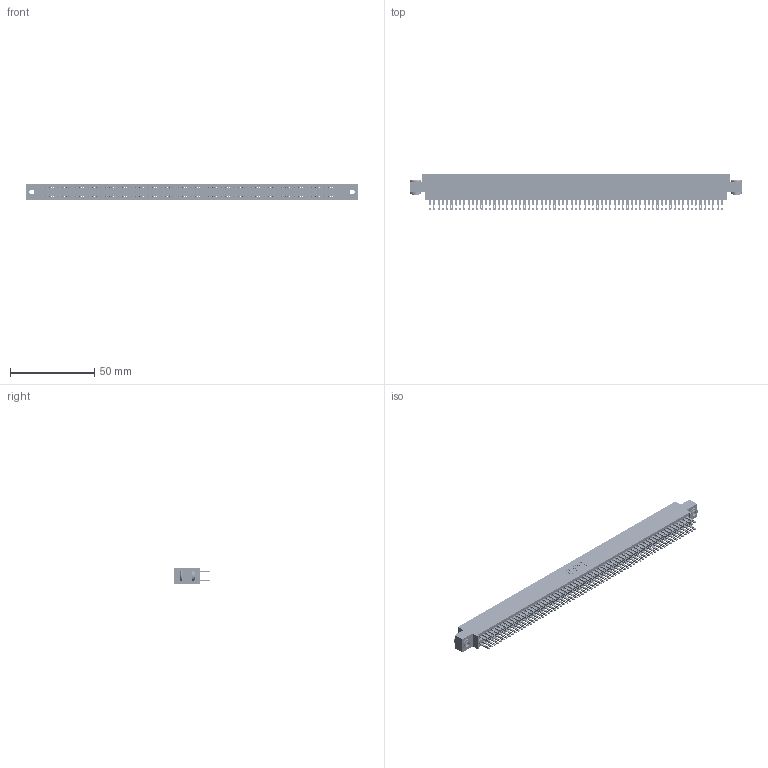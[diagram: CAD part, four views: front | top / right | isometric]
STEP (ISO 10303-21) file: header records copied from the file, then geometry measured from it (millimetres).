
FILE_DESCRIPTION (( 'STEP AP203' ), '1' );
FILE_NAME ('895-138-500-803.STEP', '2020-10-13T19:05:36', ( '' ), ( '' ), 'SwSTEP 2.0', 'SolidWorks 2020', '' );
FILE_SCHEMA (( 'CONFIG_CONTROL_DESIGN' ));
Length unit declared in the file: inch
Products named in the file (4): 845 Part_0.170 Offset - 0.156 Dia-TH; 345-292-001_345-293-100; 895-138-500-803; 345-250-002_345-250-002-102
Assembly tree (141 placements, depth 2):
  895-138-500-803
    845 Part_0.170 Offset - 0.156 Dia-TH
    345-292-001_345-293-100  x138
    345-250-002_345-250-002-102  x2
Bounding box: 196.47 x 21.51 x 9.4 mm (x, y, z)
Volume: 19663.5 mm3; surface area: 31344.8 mm2
Topology: 141 solids, 141 shells, 6516 faces, 19887 edges, 13254 vertices
Faces by surface type: plane 3820, cylinder 2688, cone 8
Entity records: 51216 total; most frequent: CARTESIAN_POINT 8535, ORIENTED_EDGE 8462, DIRECTION 7525, EDGE_CURVE 4231, VECTOR 3795, LINE 3795, VERTEX_POINT 2818, AXIS2_PLACEMENT_3D 1865
